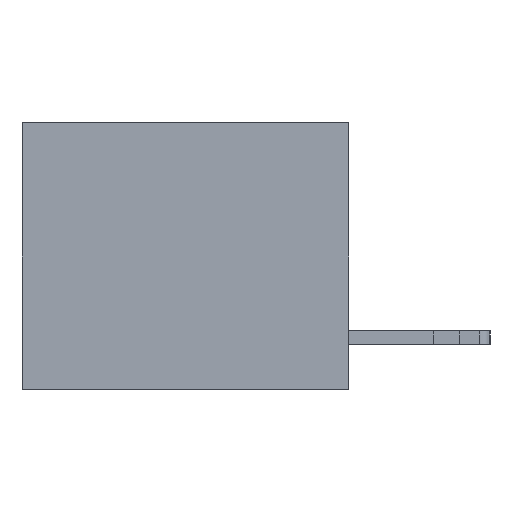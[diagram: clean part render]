
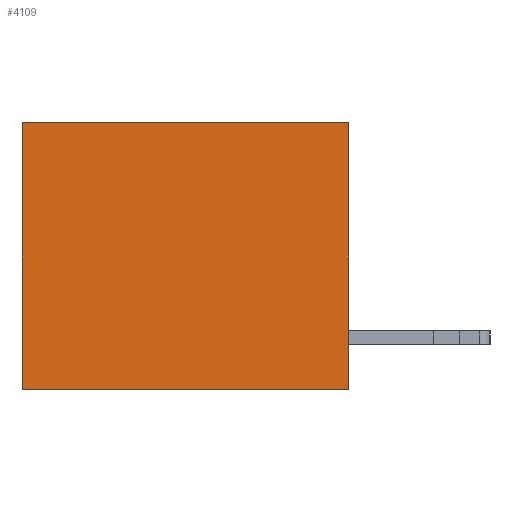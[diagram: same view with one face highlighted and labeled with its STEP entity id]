
A CAD part, left-side view. The second image highlights one B-rep face of the part: STEP entity #4109.
In plain terms, the highlighted planar face has unit normal (-1, 0, 0).
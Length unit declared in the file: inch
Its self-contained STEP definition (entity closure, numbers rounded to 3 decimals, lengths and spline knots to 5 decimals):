
#871 = VECTOR ( 'NONE', #12279, 39.37008 ) ;
#1599 = ORIENTED_EDGE ( 'NONE', *, *, #20272, .F. ) ;
#1776 = VERTEX_POINT ( 'NONE', #2846 ) ;
#1975 = EDGE_CURVE ( 'NONE', #1776, #11141, #6909, .T. ) ;
#2546 = LINE ( 'NONE', #17354, #871 ) ;
#2846 = CARTESIAN_POINT ( 'NONE',  ( 0.3165, 0.6, 0. ) ) ;
#3552 = EDGE_LOOP ( 'NONE', ( #4809, #9952, #1599, #20849 ) ) ;
#4109 = ADVANCED_FACE ( 'NONE', ( #19878 ), #22377, .F. ) ;
#4505 = DIRECTION ( 'NONE',  ( 1., 0., 0. ) ) ;
#4763 = CARTESIAN_POINT ( 'NONE',  ( 0.3165, 0., -0.49 ) ) ;
#4809 = ORIENTED_EDGE ( 'NONE', *, *, #1975, .T. ) ;
#5924 = CARTESIAN_POINT ( 'NONE',  ( 0.3165, 0., -0.49 ) ) ;
#6020 = VECTOR ( 'NONE', #14567, 39.37008 ) ;
#6558 = EDGE_CURVE ( 'NONE', #10086, #1776, #2546, .T. ) ;
#6909 = LINE ( 'NONE', #9014, #19634 ) ;
#7916 = AXIS2_PLACEMENT_3D ( 'NONE', #11634, #4505, #15248 ) ;
#9014 = CARTESIAN_POINT ( 'NONE',  ( 0.3165, 0.6, -0.49 ) ) ;
#9952 = ORIENTED_EDGE ( 'NONE', *, *, #17706, .F. ) ;
#10086 = VERTEX_POINT ( 'NONE', #13695 ) ;
#11141 = VERTEX_POINT ( 'NONE', #18444 ) ;
#11634 = CARTESIAN_POINT ( 'NONE',  ( 0.3165, 0., -0.49 ) ) ;
#11831 = VERTEX_POINT ( 'NONE', #4763 ) ;
#12044 = VECTOR ( 'NONE', #18116, 39.37008 ) ;
#12279 = DIRECTION ( 'NONE',  ( 0., 1., 0. ) ) ;
#13695 = CARTESIAN_POINT ( 'NONE',  ( 0.3165, 0., 0. ) ) ;
#14567 = DIRECTION ( 'NONE',  ( 0., 1., 0. ) ) ;
#15248 = DIRECTION ( 'NONE',  ( 0., 0., -1. ) ) ;
#15357 = LINE ( 'NONE', #5924, #12044 ) ;
#17354 = CARTESIAN_POINT ( 'NONE',  ( 0.3165, 0., 0. ) ) ;
#17706 = EDGE_CURVE ( 'NONE', #11831, #11141, #18194, .T. ) ;
#17906 = DIRECTION ( 'NONE',  ( 0., 0., -1. ) ) ;
#18116 = DIRECTION ( 'NONE',  ( 0., 0., -1. ) ) ;
#18194 = LINE ( 'NONE', #21442, #6020 ) ;
#18444 = CARTESIAN_POINT ( 'NONE',  ( 0.3165, 0.6, -0.49 ) ) ;
#19634 = VECTOR ( 'NONE', #17906, 39.37008 ) ;
#19878 = FACE_OUTER_BOUND ( 'NONE', #3552, .T. ) ;
#20272 = EDGE_CURVE ( 'NONE', #10086, #11831, #15357, .T. ) ;
#20849 = ORIENTED_EDGE ( 'NONE', *, *, #6558, .T. ) ;
#21442 = CARTESIAN_POINT ( 'NONE',  ( 0.3165, 0., -0.49 ) ) ;
#22377 = PLANE ( 'NONE',  #7916 ) ;
